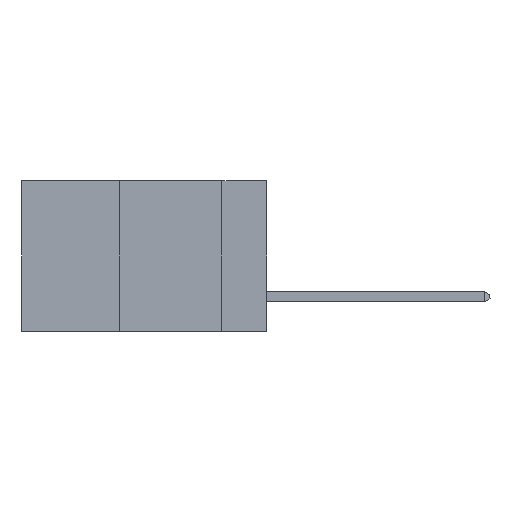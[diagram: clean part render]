
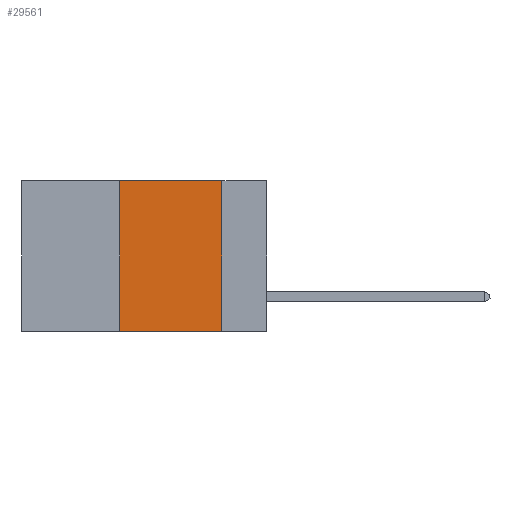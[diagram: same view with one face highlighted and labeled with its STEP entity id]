
A CAD part, left-side view. The second image highlights one B-rep face of the part: STEP entity #29561.
In plain terms, the highlighted planar face has unit normal (-1, 0, 0).
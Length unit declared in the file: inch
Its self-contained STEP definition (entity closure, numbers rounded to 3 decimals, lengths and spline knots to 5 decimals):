
#317 = CARTESIAN_POINT ( 'NONE',  ( 0., 0.6, -0.37 ) ) ;
#1015 = CARTESIAN_POINT ( 'NONE',  ( 0., 0.11, 0. ) ) ;
#1677 = ORIENTED_EDGE ( 'NONE', *, *, #17254, .T. ) ;
#1959 = ORIENTED_EDGE ( 'NONE', *, *, #23504, .F. ) ;
#2401 = ORIENTED_EDGE ( 'NONE', *, *, #31850, .F. ) ;
#3001 = VECTOR ( 'NONE', #9191, 39.37008 ) ;
#5880 = EDGE_LOOP ( 'NONE', ( #14932, #2401, #1959, #1677 ) ) ;
#6244 = CARTESIAN_POINT ( 'NONE',  ( 0., 0.36, -0.37 ) ) ;
#6632 = CARTESIAN_POINT ( 'NONE',  ( 0., 0.36, 0. ) ) ;
#6686 = CARTESIAN_POINT ( 'NONE',  ( 0., 0.11, 0. ) ) ;
#8127 = DIRECTION ( 'NONE',  ( 1., 0., 0. ) ) ;
#8908 = VECTOR ( 'NONE', #16401, 39.37008 ) ;
#9191 = DIRECTION ( 'NONE',  ( 0., 0., 1. ) ) ;
#9252 = LINE ( 'NONE', #30572, #28850 ) ;
#11819 = VERTEX_POINT ( 'NONE', #6244 ) ;
#12575 = AXIS2_PLACEMENT_3D ( 'NONE', #18349, #8127, #26037 ) ;
#13875 = VECTOR ( 'NONE', #20844, 39.37008 ) ;
#14696 = LINE ( 'NONE', #317, #13875 ) ;
#14932 = ORIENTED_EDGE ( 'NONE', *, *, #31459, .F. ) ;
#15625 = VERTEX_POINT ( 'NONE', #6686 ) ;
#16401 = DIRECTION ( 'NONE',  ( 0., 0., -1. ) ) ;
#16552 = LINE ( 'NONE', #1015, #8908 ) ;
#17254 = EDGE_CURVE ( 'NONE', #11819, #23014, #14696, .T. ) ;
#18349 = CARTESIAN_POINT ( 'NONE',  ( 0., 0.6, 0. ) ) ;
#20844 = DIRECTION ( 'NONE',  ( 0., -1., 0. ) ) ;
#20845 = VERTEX_POINT ( 'NONE', #26123 ) ;
#22666 = CARTESIAN_POINT ( 'NONE',  ( 0., 0.11, -0.37 ) ) ;
#23014 = VERTEX_POINT ( 'NONE', #22666 ) ;
#23053 = DIRECTION ( 'NONE',  ( 0., -1., 0. ) ) ;
#23399 = LINE ( 'NONE', #6632, #3001 ) ;
#23504 = EDGE_CURVE ( 'NONE', #11819, #20845, #23399, .T. ) ;
#26037 = DIRECTION ( 'NONE',  ( 0., 0., -1. ) ) ;
#26123 = CARTESIAN_POINT ( 'NONE',  ( 0., 0.36, 0. ) ) ;
#28850 = VECTOR ( 'NONE', #23053, 39.37008 ) ;
#29561 = ADVANCED_FACE ( 'NONE', ( #29922 ), #30967, .F. ) ;
#29922 = FACE_OUTER_BOUND ( 'NONE', #5880, .T. ) ;
#30572 = CARTESIAN_POINT ( 'NONE',  ( 0., 0.6, 0. ) ) ;
#30967 = PLANE ( 'NONE',  #12575 ) ;
#31459 = EDGE_CURVE ( 'NONE', #15625, #23014, #16552, .T. ) ;
#31850 = EDGE_CURVE ( 'NONE', #20845, #15625, #9252, .T. ) ;
